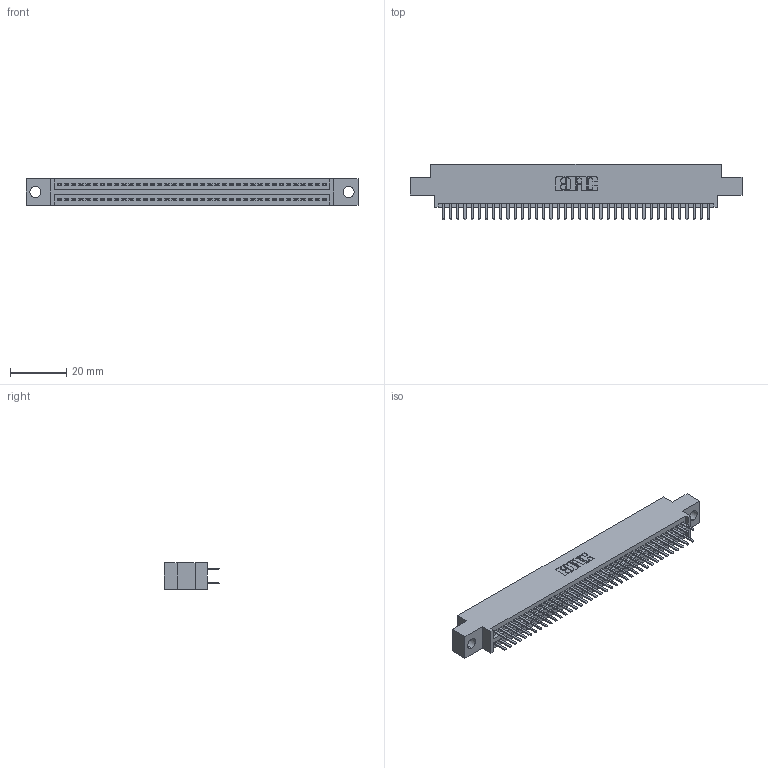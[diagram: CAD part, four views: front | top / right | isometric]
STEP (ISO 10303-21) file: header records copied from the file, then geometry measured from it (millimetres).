
FILE_DESCRIPTION (( 'STEP AP203' ), '1' );
FILE_NAME ('345-076-520-804.STEP', '2021-05-20T09:55:32', ( '' ), ( '' ), 'SwSTEP 2.0', 'SolidWorks 2020', '' );
FILE_SCHEMA (( 'CONFIG_CONTROL_DESIGN' ));
Length unit declared in the file: inch
Products named in the file (3): 345-292-001_345-293-120; 345-076-520-804; 345 Part_0.170 Offset - 0.156 Dia-TI
Assembly tree (77 placements, depth 2):
  345-076-520-804
    345 Part_0.170 Offset - 0.156 Dia-TI
    345-292-001_345-293-120  x76
Bounding box: 117.73 x 19.68 x 9.4 mm (x, y, z)
Volume: 11146.4 mm3; surface area: 16322.8 mm2
Topology: 77 solids, 77 shells, 4248 faces, 12321 edges, 8010 vertices
Faces by surface type: plane 2758, cylinder 1490
Entity records: 31019 total; most frequent: CARTESIAN_POINT 5222, ORIENTED_EDGE 5142, DIRECTION 4595, EDGE_CURVE 2571, VECTOR 2283, LINE 2283, VERTEX_POINT 1710, AXIS2_PLACEMENT_3D 1156
